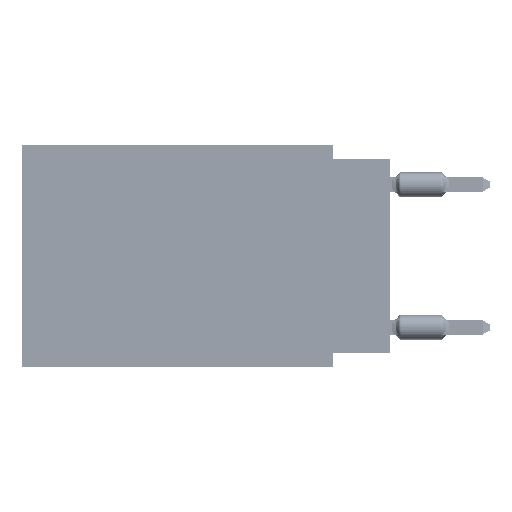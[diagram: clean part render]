
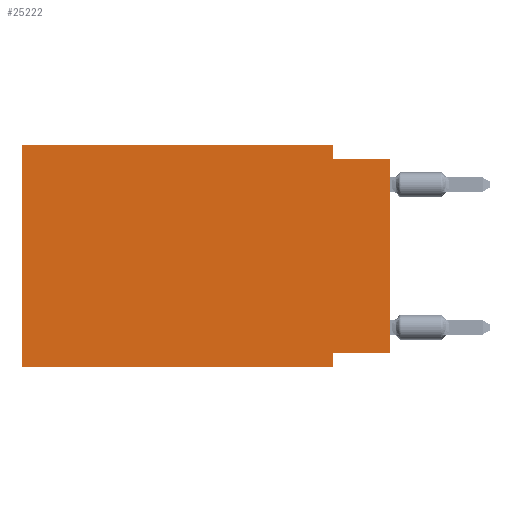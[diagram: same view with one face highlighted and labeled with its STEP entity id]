
A CAD part, left-side view. The second image highlights one B-rep face of the part: STEP entity #25222.
In plain terms, the highlighted planar face has unit normal (-1, 0, 0).
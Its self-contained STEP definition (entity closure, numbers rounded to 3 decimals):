
#1023 = EDGE_CURVE ( 'NONE', #32970, #59695, #33832, .T. ) ;
#3521 = CARTESIAN_POINT ( 'NONE',  ( 0., 0., -0.635 ) ) ;
#3689 = LINE ( 'NONE', #67546, #19212 ) ;
#5115 = VECTOR ( 'NONE', #51945, 1000. ) ;
#5454 = LINE ( 'NONE', #46189, #49467 ) ;
#6366 = EDGE_CURVE ( 'NONE', #7776, #75043, #32730, .T. ) ;
#6595 = EDGE_CURVE ( 'NONE', #32509, #7776, #12716, .T. ) ;
#7776 = VERTEX_POINT ( 'NONE', #48461 ) ;
#11158 = DIRECTION ( 'NONE',  ( 0., 0., -1. ) ) ;
#11299 = DIRECTION ( 'NONE',  ( 0., 1., 0. ) ) ;
#11321 = DIRECTION ( 'NONE',  ( 1., 0., 0. ) ) ;
#12536 = VECTOR ( 'NONE', #45028, 1000. ) ;
#12716 = LINE ( 'NONE', #64653, #5115 ) ;
#14178 = ORIENTED_EDGE ( 'NONE', *, *, #23528, .F. ) ;
#15845 = DIRECTION ( 'NONE',  ( 0., 0., 1. ) ) ;
#16323 = EDGE_CURVE ( 'NONE', #58747, #70951, #5454, .T. ) ;
#16569 = LINE ( 'NONE', #40000, #25562 ) ;
#17512 = ORIENTED_EDGE ( 'NONE', *, *, #45620, .F. ) ;
#19212 = VECTOR ( 'NONE', #38655, 1000. ) ;
#19784 = VERTEX_POINT ( 'NONE', #55749 ) ;
#21573 = EDGE_LOOP ( 'NONE', ( #41511, #54282, #36831, #17512, #34911, #52659, #23557, #14178 ) ) ;
#22858 = PLANE ( 'NONE',  #33453 ) ;
#23528 = EDGE_CURVE ( 'NONE', #19784, #32970, #56401, .T. ) ;
#23557 = ORIENTED_EDGE ( 'NONE', *, *, #1023, .F. ) ;
#25222 = ADVANCED_FACE ( 'NONE', ( #69023 ), #22858, .F. ) ;
#25562 = VECTOR ( 'NONE', #63485, 1000. ) ;
#25758 = CARTESIAN_POINT ( 'NONE',  ( 0., 16.383, -9.906 ) ) ;
#26863 = CARTESIAN_POINT ( 'NONE',  ( 0., 2.54, -9.271 ) ) ;
#30550 = CARTESIAN_POINT ( 'NONE',  ( 0., 16.383, -9.906 ) ) ;
#32509 = VERTEX_POINT ( 'NONE', #45020 ) ;
#32730 = LINE ( 'NONE', #3521, #12536 ) ;
#32970 = VERTEX_POINT ( 'NONE', #26863 ) ;
#33021 = LINE ( 'NONE', #25758, #73285 ) ;
#33453 = AXIS2_PLACEMENT_3D ( 'NONE', #58616, #11321, #33986 ) ;
#33832 = LINE ( 'NONE', #40352, #40950 ) ;
#33986 = DIRECTION ( 'NONE',  ( 0., 0., -1. ) ) ;
#34911 = ORIENTED_EDGE ( 'NONE', *, *, #16323, .F. ) ;
#36831 = ORIENTED_EDGE ( 'NONE', *, *, #6595, .F. ) ;
#38608 = CARTESIAN_POINT ( 'NONE',  ( 0., 0., -0.635 ) ) ;
#38655 = DIRECTION ( 'NONE',  ( 0., -1., 0. ) ) ;
#39072 = CARTESIAN_POINT ( 'NONE',  ( 0., 0., -9.271 ) ) ;
#40000 = CARTESIAN_POINT ( 'NONE',  ( 0., 0., 0. ) ) ;
#40352 = CARTESIAN_POINT ( 'NONE',  ( 0., 2.54, -9.906 ) ) ;
#40950 = VECTOR ( 'NONE', #11158, 1000. ) ;
#41511 = ORIENTED_EDGE ( 'NONE', *, *, #73089, .T. ) ;
#45020 = CARTESIAN_POINT ( 'NONE',  ( 0., 2.54, 0. ) ) ;
#45028 = DIRECTION ( 'NONE',  ( 0., -1., 0. ) ) ;
#45620 = EDGE_CURVE ( 'NONE', #70951, #32509, #3689, .T. ) ;
#46189 = CARTESIAN_POINT ( 'NONE',  ( 0., 16.383, 0. ) ) ;
#48461 = CARTESIAN_POINT ( 'NONE',  ( 0., 2.54, -0.635 ) ) ;
#49458 = EDGE_CURVE ( 'NONE', #58747, #59695, #33021, .T. ) ;
#49467 = VECTOR ( 'NONE', #15845, 1000. ) ;
#49988 = VECTOR ( 'NONE', #11299, 1000. ) ;
#51945 = DIRECTION ( 'NONE',  ( 0., 0., -1. ) ) ;
#52659 = ORIENTED_EDGE ( 'NONE', *, *, #49458, .T. ) ;
#54282 = ORIENTED_EDGE ( 'NONE', *, *, #6366, .F. ) ;
#55749 = CARTESIAN_POINT ( 'NONE',  ( 0., 0., -9.271 ) ) ;
#56401 = LINE ( 'NONE', #39072, #49988 ) ;
#58616 = CARTESIAN_POINT ( 'NONE',  ( 0., 16.383, 0. ) ) ;
#58747 = VERTEX_POINT ( 'NONE', #30550 ) ;
#59695 = VERTEX_POINT ( 'NONE', #68320 ) ;
#63485 = DIRECTION ( 'NONE',  ( 0., 0., 1. ) ) ;
#64653 = CARTESIAN_POINT ( 'NONE',  ( 0., 2.54, 0. ) ) ;
#65328 = CARTESIAN_POINT ( 'NONE',  ( 0., 16.383, 0. ) ) ;
#67546 = CARTESIAN_POINT ( 'NONE',  ( 0., 16.383, 0. ) ) ;
#68320 = CARTESIAN_POINT ( 'NONE',  ( 0., 2.54, -9.906 ) ) ;
#69023 = FACE_OUTER_BOUND ( 'NONE', #21573, .T. ) ;
#70951 = VERTEX_POINT ( 'NONE', #65328 ) ;
#72685 = DIRECTION ( 'NONE',  ( 0., -1., 0. ) ) ;
#73089 = EDGE_CURVE ( 'NONE', #19784, #75043, #16569, .T. ) ;
#73285 = VECTOR ( 'NONE', #72685, 1000. ) ;
#75043 = VERTEX_POINT ( 'NONE', #38608 ) ;
